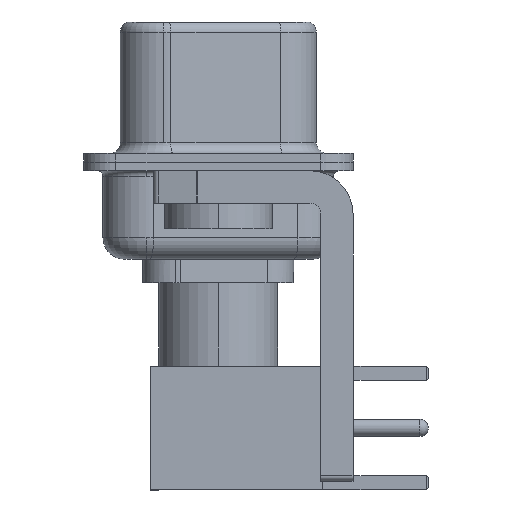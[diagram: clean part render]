
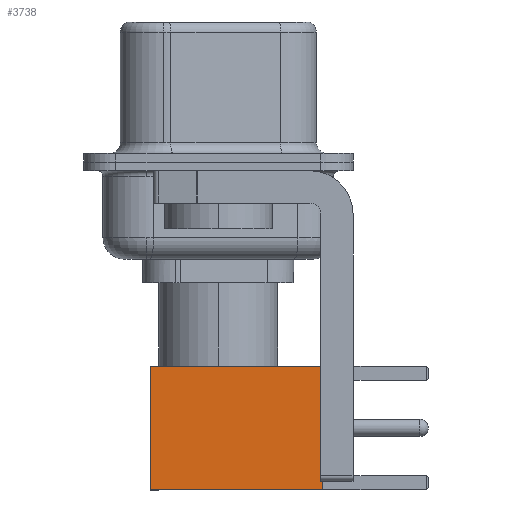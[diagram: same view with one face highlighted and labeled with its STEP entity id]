
A CAD part, left-side view. The second image highlights one B-rep face of the part: STEP entity #3738.
In plain terms, the highlighted face is planar.
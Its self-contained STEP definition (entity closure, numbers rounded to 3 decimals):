
#393 = VECTOR ( 'NONE', #14747, 1000. ) ;
#1358 = VECTOR ( 'NONE', #1626, 1000. ) ;
#1626 = DIRECTION ( 'NONE',  ( 0., 0., -1. ) ) ;
#1661 = EDGE_CURVE ( 'NONE', #10219, #3195, #8010, .T. ) ;
#1929 = LINE ( 'NONE', #4324, #393 ) ;
#2218 = CARTESIAN_POINT ( 'NONE',  ( -2.875, 2.875, 0. ) ) ;
#2450 = EDGE_CURVE ( 'NONE', #6873, #6700, #14798, .T. ) ;
#3195 = VERTEX_POINT ( 'NONE', #14207 ) ;
#3738 = ADVANCED_FACE ( 'NONE', ( #8091 ), #14612, .T. ) ;
#3750 = EDGE_LOOP ( 'NONE', ( #13907, #7408, #5786, #7913 ) ) ;
#4324 = CARTESIAN_POINT ( 'NONE',  ( 0., 2.875, 8. ) ) ;
#4366 = EDGE_CURVE ( 'NONE', #10219, #6873, #1929, .T. ) ;
#5736 = VECTOR ( 'NONE', #9062, 1000. ) ;
#5786 = ORIENTED_EDGE ( 'NONE', *, *, #2450, .F. ) ;
#6700 = VERTEX_POINT ( 'NONE', #2218 ) ;
#6726 = CARTESIAN_POINT ( 'NONE',  ( 2.875, 2.875, 0. ) ) ;
#6802 = DIRECTION ( 'NONE',  ( 0., 1., 0. ) ) ;
#6873 = VERTEX_POINT ( 'NONE', #10039 ) ;
#7408 = ORIENTED_EDGE ( 'NONE', *, *, #10142, .T. ) ;
#7699 = CARTESIAN_POINT ( 'NONE',  ( 0., 2.875, 0. ) ) ;
#7913 = ORIENTED_EDGE ( 'NONE', *, *, #4366, .F. ) ;
#8010 = LINE ( 'NONE', #11990, #1358 ) ;
#8091 = FACE_OUTER_BOUND ( 'NONE', #3750, .T. ) ;
#8529 = VECTOR ( 'NONE', #12352, 1000. ) ;
#8624 = CARTESIAN_POINT ( 'NONE',  ( -2.875, 2.875, 0. ) ) ;
#9062 = DIRECTION ( 'NONE',  ( -1., 0., 0. ) ) ;
#10039 = CARTESIAN_POINT ( 'NONE',  ( -2.875, 2.875, 8. ) ) ;
#10142 = EDGE_CURVE ( 'NONE', #3195, #6700, #15679, .T. ) ;
#10219 = VERTEX_POINT ( 'NONE', #10582 ) ;
#10582 = CARTESIAN_POINT ( 'NONE',  ( 2.875, 2.875, 8. ) ) ;
#11674 = AXIS2_PLACEMENT_3D ( 'NONE', #6726, #6802, #11906 ) ;
#11906 = DIRECTION ( 'NONE',  ( 0., 0., 1. ) ) ;
#11990 = CARTESIAN_POINT ( 'NONE',  ( 2.875, 2.875, 0. ) ) ;
#12352 = DIRECTION ( 'NONE',  ( 0., 0., -1. ) ) ;
#13907 = ORIENTED_EDGE ( 'NONE', *, *, #1661, .T. ) ;
#14207 = CARTESIAN_POINT ( 'NONE',  ( 2.875, 2.875, 0. ) ) ;
#14612 = PLANE ( 'NONE',  #11674 ) ;
#14747 = DIRECTION ( 'NONE',  ( -1., 0., 0. ) ) ;
#14798 = LINE ( 'NONE', #8624, #8529 ) ;
#15679 = LINE ( 'NONE', #7699, #5736 ) ;
